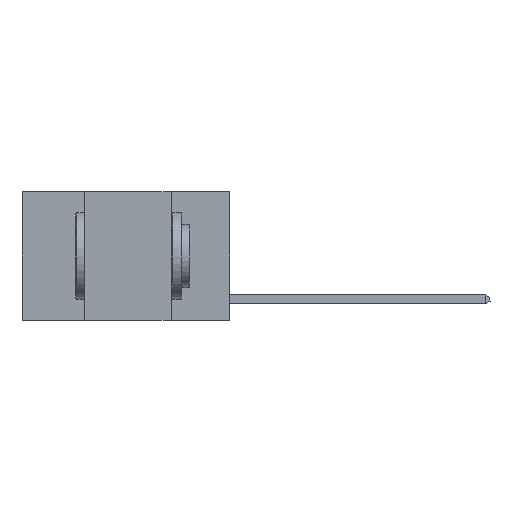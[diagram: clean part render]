
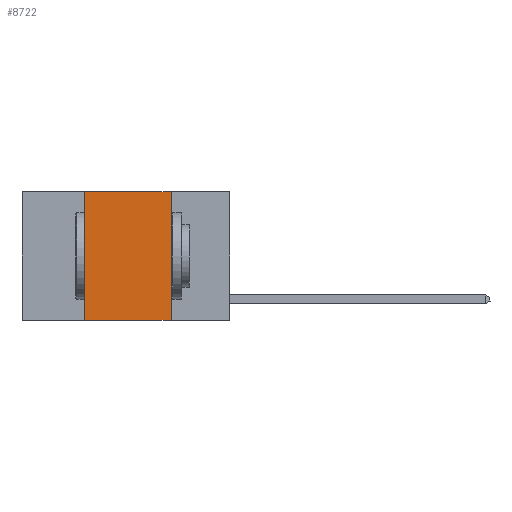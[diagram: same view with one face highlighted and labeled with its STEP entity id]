
A CAD part, left-side view. The second image highlights one B-rep face of the part: STEP entity #8722.
In plain terms, the highlighted planar face has unit normal (-1, 0, 0).
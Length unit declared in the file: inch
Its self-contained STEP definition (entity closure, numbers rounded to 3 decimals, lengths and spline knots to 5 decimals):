
#121 = VERTEX_POINT ( 'NONE', #3041 ) ;
#161 = EDGE_CURVE ( 'NONE', #4379, #13329, #3092, .T. ) ;
#200 = CARTESIAN_POINT ( 'NONE',  ( 0., 0.42, -0.37 ) ) ;
#618 = ORIENTED_EDGE ( 'NONE', *, *, #13267, .F. ) ;
#1012 = EDGE_CURVE ( 'NONE', #4379, #1826, #9780, .T. ) ;
#1020 = ORIENTED_EDGE ( 'NONE', *, *, #161, .T. ) ;
#1644 = CARTESIAN_POINT ( 'NONE',  ( 0., 0.6, 0. ) ) ;
#1826 = VERTEX_POINT ( 'NONE', #10679 ) ;
#2102 = LINE ( 'NONE', #7415, #11750 ) ;
#3041 = CARTESIAN_POINT ( 'NONE',  ( 0., 0.17, 0. ) ) ;
#3092 = LINE ( 'NONE', #6785, #9007 ) ;
#3868 = DIRECTION ( 'NONE',  ( 0., 0., 1. ) ) ;
#4379 = VERTEX_POINT ( 'NONE', #200 ) ;
#5398 = PLANE ( 'NONE',  #7731 ) ;
#5969 = DIRECTION ( 'NONE',  ( 0., -1., 0. ) ) ;
#6024 = VECTOR ( 'NONE', #3868, 39.37008 ) ;
#6656 = DIRECTION ( 'NONE',  ( 0., 0., -1. ) ) ;
#6685 = CARTESIAN_POINT ( 'NONE',  ( 0., 0.6, 0. ) ) ;
#6785 = CARTESIAN_POINT ( 'NONE',  ( 0., 0.6, -0.37 ) ) ;
#6858 = CARTESIAN_POINT ( 'NONE',  ( 0., 0.42, 0. ) ) ;
#6877 = ORIENTED_EDGE ( 'NONE', *, *, #7721, .F. ) ;
#7415 = CARTESIAN_POINT ( 'NONE',  ( 0., 0.17, 0. ) ) ;
#7721 = EDGE_CURVE ( 'NONE', #121, #13329, #2102, .T. ) ;
#7731 = AXIS2_PLACEMENT_3D ( 'NONE', #1644, #14174, #6656 ) ;
#7950 = DIRECTION ( 'NONE',  ( 0., -1., 0. ) ) ;
#8722 = ADVANCED_FACE ( 'NONE', ( #10121 ), #5398, .F. ) ;
#9007 = VECTOR ( 'NONE', #5969, 39.37008 ) ;
#9191 = LINE ( 'NONE', #6685, #15807 ) ;
#9704 = EDGE_LOOP ( 'NONE', ( #6877, #618, #10634, #1020 ) ) ;
#9780 = LINE ( 'NONE', #6858, #6024 ) ;
#10028 = DIRECTION ( 'NONE',  ( 0., 0., -1. ) ) ;
#10121 = FACE_OUTER_BOUND ( 'NONE', #9704, .T. ) ;
#10634 = ORIENTED_EDGE ( 'NONE', *, *, #1012, .F. ) ;
#10679 = CARTESIAN_POINT ( 'NONE',  ( 0., 0.42, 0. ) ) ;
#11750 = VECTOR ( 'NONE', #10028, 39.37008 ) ;
#13063 = CARTESIAN_POINT ( 'NONE',  ( 0., 0.17, -0.37 ) ) ;
#13267 = EDGE_CURVE ( 'NONE', #1826, #121, #9191, .T. ) ;
#13329 = VERTEX_POINT ( 'NONE', #13063 ) ;
#14174 = DIRECTION ( 'NONE',  ( 1., 0., 0. ) ) ;
#15807 = VECTOR ( 'NONE', #7950, 39.37008 ) ;
